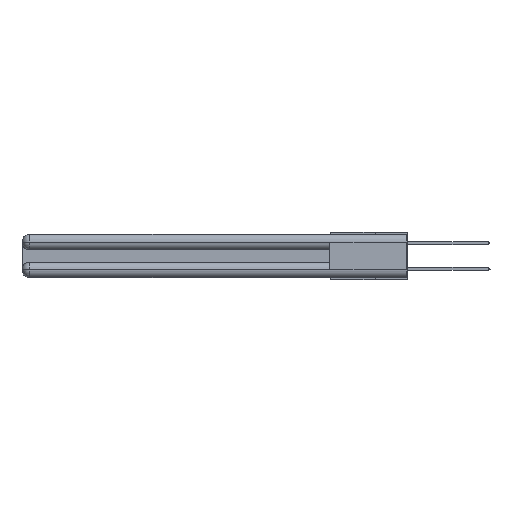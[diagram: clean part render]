
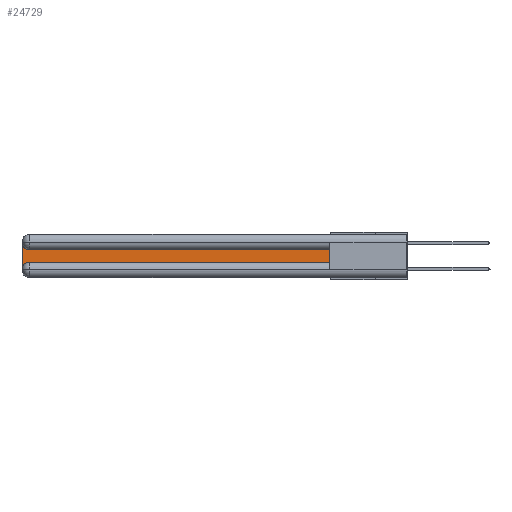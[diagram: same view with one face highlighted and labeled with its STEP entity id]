
A CAD part, left-side view. The second image highlights one B-rep face of the part: STEP entity #24729.
In plain terms, the highlighted planar face has unit normal (-1, 0, 0).
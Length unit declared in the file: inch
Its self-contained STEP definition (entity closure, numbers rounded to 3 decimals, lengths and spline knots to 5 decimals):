
#6 = LINE ( 'NONE', #17825, #10462 ) ;
#47 = ORIENTED_EDGE ( 'NONE', *, *, #16335, .T. ) ;
#671 = CIRCLE ( 'NONE', #27283, 0.06 ) ;
#775 = DIRECTION ( 'NONE',  ( 1., 0., 0. ) ) ;
#1091 = ORIENTED_EDGE ( 'NONE', *, *, #12407, .T. ) ;
#1332 = FACE_OUTER_BOUND ( 'NONE', #8630, .T. ) ;
#1630 = CARTESIAN_POINT ( 'NONE',  ( 0.075, 3., -0.2175 ) ) ;
#2406 = CARTESIAN_POINT ( 'NONE',  ( 0.075, 0.6, -0.2175 ) ) ;
#2660 = ORIENTED_EDGE ( 'NONE', *, *, #12475, .T. ) ;
#4048 = VECTOR ( 'NONE', #4682, 39.37008 ) ;
#4682 = DIRECTION ( 'NONE',  ( 0., -1., 0. ) ) ;
#4749 = LINE ( 'NONE', #2406, #4048 ) ;
#5141 = AXIS2_PLACEMENT_3D ( 'NONE', #25819, #12540, #28049 ) ;
#6061 = DIRECTION ( 'NONE',  ( 1., 0., 0. ) ) ;
#6799 = DIRECTION ( 'NONE',  ( 0., 0., 1. ) ) ;
#7458 = CARTESIAN_POINT ( 'NONE',  ( 0.075, 0.6, -0.2175 ) ) ;
#7634 = VECTOR ( 'NONE', #15041, 39.37008 ) ;
#8630 = EDGE_LOOP ( 'NONE', ( #47, #18001, #2660, #1091, #18541, #27009 ) ) ;
#8632 = CARTESIAN_POINT ( 'NONE',  ( 0.075, 3., -0.2775 ) ) ;
#9708 = CARTESIAN_POINT ( 'NONE',  ( 0.075, 2.94, -0.1225 ) ) ;
#10308 = PLANE ( 'NONE',  #5141 ) ;
#10462 = VECTOR ( 'NONE', #6799, 39.37008 ) ;
#11024 = EDGE_CURVE ( 'NONE', #18923, #17693, #6, .T. ) ;
#11947 = LINE ( 'NONE', #18987, #23041 ) ;
#12407 = EDGE_CURVE ( 'NONE', #19072, #22517, #671, .T. ) ;
#12475 = EDGE_CURVE ( 'NONE', #12527, #19072, #26022, .T. ) ;
#12527 = VERTEX_POINT ( 'NONE', #22727 ) ;
#12540 = DIRECTION ( 'NONE',  ( 1., 0., 0. ) ) ;
#12752 = DIRECTION ( 'NONE',  ( 0., 0., -1. ) ) ;
#13928 = EDGE_CURVE ( 'NONE', #24905, #12527, #21060, .T. ) ;
#14016 = CARTESIAN_POINT ( 'NONE',  ( 0.075, 2.94, -0.2775 ) ) ;
#15041 = DIRECTION ( 'NONE',  ( 0., 0., -1. ) ) ;
#16304 = DIRECTION ( 'NONE',  ( 0., 0., -1. ) ) ;
#16335 = EDGE_CURVE ( 'NONE', #17693, #24905, #11947, .T. ) ;
#17018 = DIRECTION ( 'NONE',  ( 0., 1., 0. ) ) ;
#17693 = VERTEX_POINT ( 'NONE', #27079 ) ;
#17825 = CARTESIAN_POINT ( 'NONE',  ( 0.075, 0.6, -0.2175 ) ) ;
#17989 = AXIS2_PLACEMENT_3D ( 'NONE', #19426, #6061, #12752 ) ;
#18001 = ORIENTED_EDGE ( 'NONE', *, *, #13928, .T. ) ;
#18541 = ORIENTED_EDGE ( 'NONE', *, *, #26948, .T. ) ;
#18923 = VERTEX_POINT ( 'NONE', #7458 ) ;
#18987 = CARTESIAN_POINT ( 'NONE',  ( 0.075, 0.6, -0.1225 ) ) ;
#19072 = VERTEX_POINT ( 'NONE', #8632 ) ;
#19426 = CARTESIAN_POINT ( 'NONE',  ( 0.075, 2.94, -0.0625 ) ) ;
#21060 = CIRCLE ( 'NONE', #17989, 0.06 ) ;
#22517 = VERTEX_POINT ( 'NONE', #22901 ) ;
#22727 = CARTESIAN_POINT ( 'NONE',  ( 0.075, 3., -0.0625 ) ) ;
#22901 = CARTESIAN_POINT ( 'NONE',  ( 0.075, 2.94, -0.2175 ) ) ;
#23041 = VECTOR ( 'NONE', #17018, 39.37008 ) ;
#24729 = ADVANCED_FACE ( 'NONE', ( #1332 ), #10308, .F. ) ;
#24905 = VERTEX_POINT ( 'NONE', #9708 ) ;
#25819 = CARTESIAN_POINT ( 'NONE',  ( 0.075, 3., -0.1225 ) ) ;
#26022 = LINE ( 'NONE', #1630, #7634 ) ;
#26948 = EDGE_CURVE ( 'NONE', #22517, #18923, #4749, .T. ) ;
#27009 = ORIENTED_EDGE ( 'NONE', *, *, #11024, .T. ) ;
#27079 = CARTESIAN_POINT ( 'NONE',  ( 0.075, 0.6, -0.1225 ) ) ;
#27283 = AXIS2_PLACEMENT_3D ( 'NONE', #14016, #775, #16304 ) ;
#28049 = DIRECTION ( 'NONE',  ( 0., 0., -1. ) ) ;
